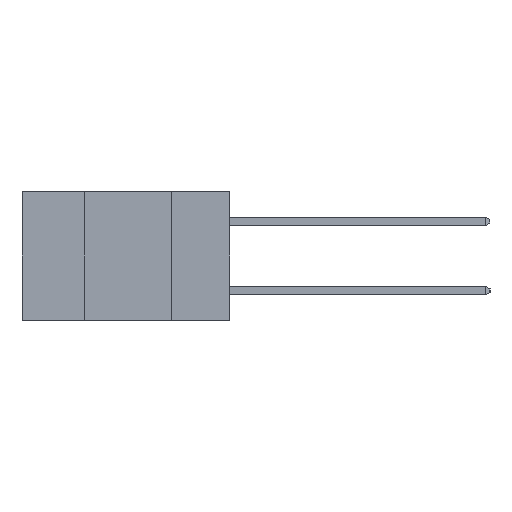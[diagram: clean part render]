
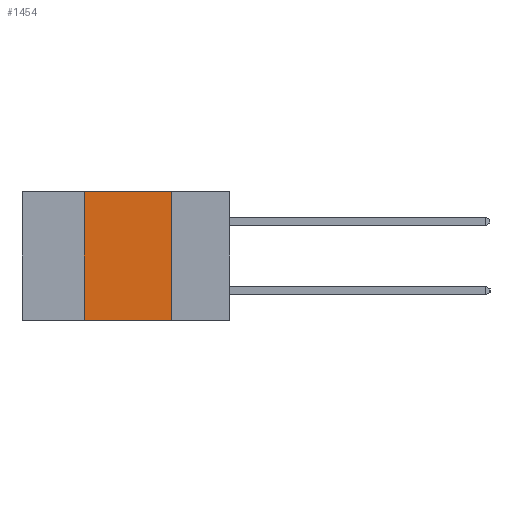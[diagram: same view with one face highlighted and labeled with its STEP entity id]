
A CAD part, left-side view. The second image highlights one B-rep face of the part: STEP entity #1454.
In plain terms, the highlighted planar face has unit normal (-1, 0, 0).
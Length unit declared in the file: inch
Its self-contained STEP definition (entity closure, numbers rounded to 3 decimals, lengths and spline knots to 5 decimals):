
#796 = EDGE_CURVE ( 'NONE', #12150, #12802, #10036, .T. ) ;
#1045 = VECTOR ( 'NONE', #18982, 39.37008 ) ;
#1454 = ADVANCED_FACE ( 'NONE', ( #15994 ), #11859, .F. ) ;
#2295 = DIRECTION ( 'NONE',  ( 1., 0., 0. ) ) ;
#4056 = CARTESIAN_POINT ( 'NONE',  ( 0., 0.17, -0.37 ) ) ;
#5248 = EDGE_CURVE ( 'NONE', #12150, #6160, #17501, .T. ) ;
#5419 = ORIENTED_EDGE ( 'NONE', *, *, #796, .F. ) ;
#5686 = DIRECTION ( 'NONE',  ( 0., 0., -1. ) ) ;
#6116 = VERTEX_POINT ( 'NONE', #11440 ) ;
#6160 = VERTEX_POINT ( 'NONE', #9957 ) ;
#6689 = VECTOR ( 'NONE', #5686, 39.37008 ) ;
#6845 = DIRECTION ( 'NONE',  ( 0., -1., 0. ) ) ;
#7712 = EDGE_CURVE ( 'NONE', #6116, #6160, #10910, .T. ) ;
#7858 = CARTESIAN_POINT ( 'NONE',  ( 0., 0.6, -0.37 ) ) ;
#8544 = DIRECTION ( 'NONE',  ( 0., 0., 1. ) ) ;
#8850 = ORIENTED_EDGE ( 'NONE', *, *, #11971, .F. ) ;
#9351 = VECTOR ( 'NONE', #6845, 39.37008 ) ;
#9957 = CARTESIAN_POINT ( 'NONE',  ( 0., 0.17, -0.37 ) ) ;
#10036 = LINE ( 'NONE', #18063, #14781 ) ;
#10518 = CARTESIAN_POINT ( 'NONE',  ( 0., 0.42, -0.37 ) ) ;
#10910 = LINE ( 'NONE', #4056, #6689 ) ;
#11440 = CARTESIAN_POINT ( 'NONE',  ( 0., 0.17, 0. ) ) ;
#11589 = CARTESIAN_POINT ( 'NONE',  ( 0., 0.6, 0. ) ) ;
#11859 = PLANE ( 'NONE',  #18300 ) ;
#11971 = EDGE_CURVE ( 'NONE', #12802, #6116, #18320, .T. ) ;
#12150 = VERTEX_POINT ( 'NONE', #10518 ) ;
#12802 = VERTEX_POINT ( 'NONE', #16965 ) ;
#13389 = CARTESIAN_POINT ( 'NONE',  ( 0., 0.6, 0. ) ) ;
#13458 = DIRECTION ( 'NONE',  ( 0., 0., -1. ) ) ;
#13464 = EDGE_LOOP ( 'NONE', ( #18146, #8850, #5419, #14483 ) ) ;
#14483 = ORIENTED_EDGE ( 'NONE', *, *, #5248, .T. ) ;
#14781 = VECTOR ( 'NONE', #8544, 39.37008 ) ;
#15994 = FACE_OUTER_BOUND ( 'NONE', #13464, .T. ) ;
#16965 = CARTESIAN_POINT ( 'NONE',  ( 0., 0.42, 0. ) ) ;
#17501 = LINE ( 'NONE', #7858, #1045 ) ;
#18063 = CARTESIAN_POINT ( 'NONE',  ( 0., 0.42, -0.37 ) ) ;
#18146 = ORIENTED_EDGE ( 'NONE', *, *, #7712, .F. ) ;
#18300 = AXIS2_PLACEMENT_3D ( 'NONE', #13389, #2295, #13458 ) ;
#18320 = LINE ( 'NONE', #11589, #9351 ) ;
#18982 = DIRECTION ( 'NONE',  ( 0., -1., 0. ) ) ;
